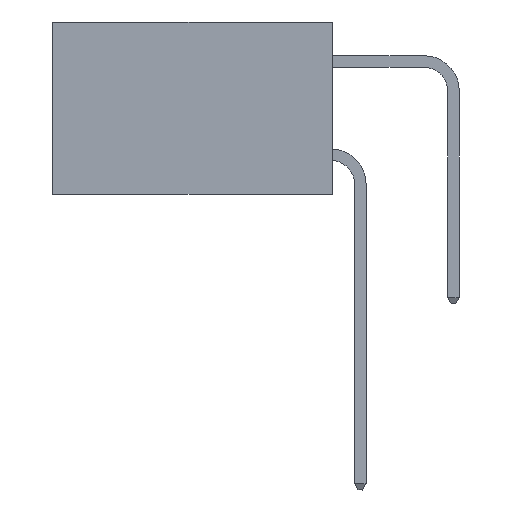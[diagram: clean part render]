
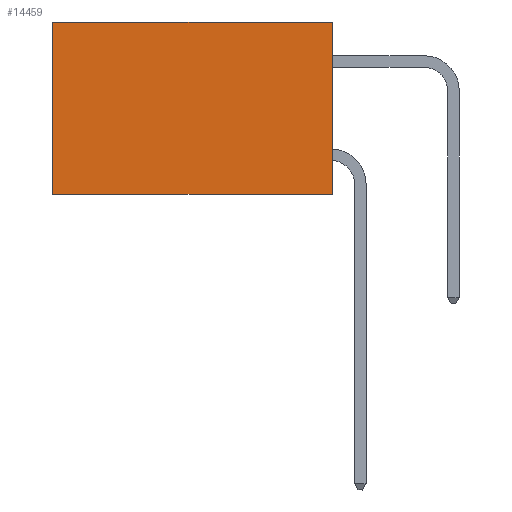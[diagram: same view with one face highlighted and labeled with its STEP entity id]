
A CAD part, left-side view. The second image highlights one B-rep face of the part: STEP entity #14459.
In plain terms, the highlighted planar face has unit normal (-1, 0, 0).
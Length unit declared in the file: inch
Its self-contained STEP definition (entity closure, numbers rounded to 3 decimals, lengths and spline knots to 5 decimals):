
#427 = LINE ( 'NONE', #5881, #15470 ) ;
#1581 = ORIENTED_EDGE ( 'NONE', *, *, #5514, .F. ) ;
#2991 = VERTEX_POINT ( 'NONE', #17505 ) ;
#3152 = LINE ( 'NONE', #7409, #3968 ) ;
#3456 = AXIS2_PLACEMENT_3D ( 'NONE', #6570, #12204, #5191 ) ;
#3968 = VECTOR ( 'NONE', #4451, 39.37008 ) ;
#4060 = ORIENTED_EDGE ( 'NONE', *, *, #10168, .T. ) ;
#4451 = DIRECTION ( 'NONE',  ( 0., 0., -1. ) ) ;
#4569 = CARTESIAN_POINT ( 'NONE',  ( 0.2615, 0., 0. ) ) ;
#5089 = VERTEX_POINT ( 'NONE', #11806 ) ;
#5191 = DIRECTION ( 'NONE',  ( 0., 0., -1. ) ) ;
#5514 = EDGE_CURVE ( 'NONE', #5089, #2991, #427, .T. ) ;
#5881 = CARTESIAN_POINT ( 'NONE',  ( 0.2615, 0., -0.37 ) ) ;
#5912 = VERTEX_POINT ( 'NONE', #10185 ) ;
#6570 = CARTESIAN_POINT ( 'NONE',  ( 0.2615, 0., -0.37 ) ) ;
#6612 = CARTESIAN_POINT ( 'NONE',  ( 0.2615, 0.6, 0. ) ) ;
#7409 = CARTESIAN_POINT ( 'NONE',  ( 0.2615, 0.6, -0.37 ) ) ;
#7437 = LINE ( 'NONE', #15531, #12070 ) ;
#7543 = DIRECTION ( 'NONE',  ( 0., 1., 0. ) ) ;
#8558 = VERTEX_POINT ( 'NONE', #6612 ) ;
#8631 = DIRECTION ( 'NONE',  ( 0., 1., 0. ) ) ;
#9252 = PLANE ( 'NONE',  #3456 ) ;
#10168 = EDGE_CURVE ( 'NONE', #8558, #2991, #3152, .T. ) ;
#10185 = CARTESIAN_POINT ( 'NONE',  ( 0.2615, 0., 0. ) ) ;
#10453 = EDGE_LOOP ( 'NONE', ( #4060, #1581, #15371, #11698 ) ) ;
#10483 = VECTOR ( 'NONE', #8631, 39.37008 ) ;
#11698 = ORIENTED_EDGE ( 'NONE', *, *, #12836, .T. ) ;
#11806 = CARTESIAN_POINT ( 'NONE',  ( 0.2615, 0., -0.37 ) ) ;
#12070 = VECTOR ( 'NONE', #12877, 39.37008 ) ;
#12204 = DIRECTION ( 'NONE',  ( 1., 0., 0. ) ) ;
#12836 = EDGE_CURVE ( 'NONE', #5912, #8558, #14246, .T. ) ;
#12877 = DIRECTION ( 'NONE',  ( 0., 0., -1. ) ) ;
#14246 = LINE ( 'NONE', #4569, #10483 ) ;
#14459 = ADVANCED_FACE ( 'NONE', ( #16278 ), #9252, .F. ) ;
#15371 = ORIENTED_EDGE ( 'NONE', *, *, #17435, .F. ) ;
#15470 = VECTOR ( 'NONE', #7543, 39.37008 ) ;
#15531 = CARTESIAN_POINT ( 'NONE',  ( 0.2615, 0., -0.37 ) ) ;
#16278 = FACE_OUTER_BOUND ( 'NONE', #10453, .T. ) ;
#17435 = EDGE_CURVE ( 'NONE', #5912, #5089, #7437, .T. ) ;
#17505 = CARTESIAN_POINT ( 'NONE',  ( 0.2615, 0.6, -0.37 ) ) ;
